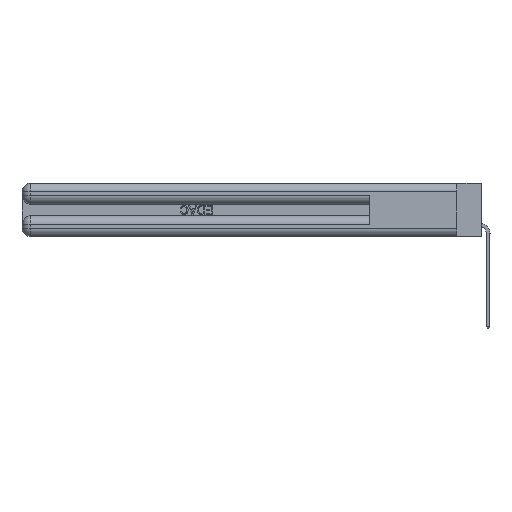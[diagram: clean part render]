
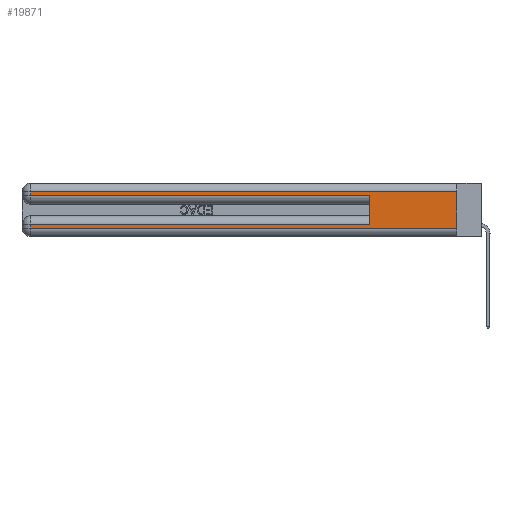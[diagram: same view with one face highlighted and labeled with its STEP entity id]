
A CAD part, left-side view. The second image highlights one B-rep face of the part: STEP entity #19871.
In plain terms, the highlighted planar face has unit normal (-1, 0, 0).
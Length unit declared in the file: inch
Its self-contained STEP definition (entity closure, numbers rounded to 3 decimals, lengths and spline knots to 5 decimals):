
#393 = FACE_OUTER_BOUND ( 'NONE', #48717, .T. ) ;
#705 = DIRECTION ( 'NONE',  ( 0., 0., -1. ) ) ;
#800 = CARTESIAN_POINT ( 'NONE',  ( 0., 0., 0.31 ) ) ;
#820 = CARTESIAN_POINT ( 'NONE',  ( 0., 2.94, 0.085 ) ) ;
#1202 = DIRECTION ( 'NONE',  ( 0., -1., 0. ) ) ;
#2137 = CARTESIAN_POINT ( 'NONE',  ( 0., 0.6, 0.145 ) ) ;
#3164 = LINE ( 'NONE', #20812, #43230 ) ;
#6102 = EDGE_CURVE ( 'NONE', #22808, #16744, #39163, .T. ) ;
#6666 = CARTESIAN_POINT ( 'NONE',  ( 0., 0.6, 0.085 ) ) ;
#9406 = LINE ( 'NONE', #800, #34781 ) ;
#10379 = DIRECTION ( 'NONE',  ( 0., 0., 1. ) ) ;
#10628 = VERTEX_POINT ( 'NONE', #6666 ) ;
#11067 = CARTESIAN_POINT ( 'NONE',  ( 0., 0., 0.06 ) ) ;
#11150 = VERTEX_POINT ( 'NONE', #13514 ) ;
#11471 = VECTOR ( 'NONE', #31491, 39.37008 ) ;
#12427 = ORIENTED_EDGE ( 'NONE', *, *, #43336, .T. ) ;
#12521 = DIRECTION ( 'NONE',  ( 0., 1., 0. ) ) ;
#12815 = VERTEX_POINT ( 'NONE', #41090 ) ;
#13514 = CARTESIAN_POINT ( 'NONE',  ( 0., 0., 0.06 ) ) ;
#13626 = DIRECTION ( 'NONE',  ( 0., 0., -1. ) ) ;
#14155 = VERTEX_POINT ( 'NONE', #41047 ) ;
#14516 = CARTESIAN_POINT ( 'NONE',  ( 0., 0., 0.085 ) ) ;
#16612 = CARTESIAN_POINT ( 'NONE',  ( 0., 2.94, 0.285 ) ) ;
#16744 = VERTEX_POINT ( 'NONE', #16612 ) ;
#17571 = ORIENTED_EDGE ( 'NONE', *, *, #6102, .T. ) ;
#17596 = EDGE_CURVE ( 'NONE', #12815, #11150, #41905, .T. ) ;
#19658 = VERTEX_POINT ( 'NONE', #820 ) ;
#19871 = ADVANCED_FACE ( 'NONE', ( #393 ), #37093, .F. ) ;
#20070 = EDGE_CURVE ( 'NONE', #19658, #14155, #26287, .T. ) ;
#20812 = CARTESIAN_POINT ( 'NONE',  ( 0., 0., 0.285 ) ) ;
#22075 = EDGE_CURVE ( 'NONE', #10628, #43003, #44084, .T. ) ;
#22808 = VERTEX_POINT ( 'NONE', #40728 ) ;
#23227 = LINE ( 'NONE', #11067, #11471 ) ;
#25273 = VECTOR ( 'NONE', #30779, 39.37008 ) ;
#25377 = AXIS2_PLACEMENT_3D ( 'NONE', #49376, #46627, #34970 ) ;
#26287 = LINE ( 'NONE', #43594, #35593 ) ;
#27361 = VECTOR ( 'NONE', #13626, 39.37008 ) ;
#28286 = CARTESIAN_POINT ( 'NONE',  ( 0., 0.6, 0.285 ) ) ;
#28544 = DIRECTION ( 'NONE',  ( 0., 0., -1. ) ) ;
#29983 = ORIENTED_EDGE ( 'NONE', *, *, #34558, .T. ) ;
#30628 = ORIENTED_EDGE ( 'NONE', *, *, #32607, .T. ) ;
#30713 = VECTOR ( 'NONE', #28544, 39.37008 ) ;
#30779 = DIRECTION ( 'NONE',  ( 0., 1., 0. ) ) ;
#31491 = DIRECTION ( 'NONE',  ( 0., -1., 0. ) ) ;
#31567 = ORIENTED_EDGE ( 'NONE', *, *, #45541, .T. ) ;
#32607 = EDGE_CURVE ( 'NONE', #10628, #19658, #50708, .T. ) ;
#33858 = CARTESIAN_POINT ( 'NONE',  ( 0., 2.94, 0.37 ) ) ;
#34558 = EDGE_CURVE ( 'NONE', #14155, #11150, #23227, .T. ) ;
#34781 = VECTOR ( 'NONE', #12521, 39.37008 ) ;
#34970 = DIRECTION ( 'NONE',  ( 0., 0., -1. ) ) ;
#35139 = ORIENTED_EDGE ( 'NONE', *, *, #22075, .F. ) ;
#35593 = VECTOR ( 'NONE', #705, 39.37008 ) ;
#35951 = ORIENTED_EDGE ( 'NONE', *, *, #17596, .F. ) ;
#37093 = PLANE ( 'NONE',  #25377 ) ;
#37314 = ORIENTED_EDGE ( 'NONE', *, *, #20070, .T. ) ;
#39163 = LINE ( 'NONE', #33858, #27361 ) ;
#40189 = CARTESIAN_POINT ( 'NONE',  ( 0., 0., 0.37 ) ) ;
#40728 = CARTESIAN_POINT ( 'NONE',  ( 0., 2.94, 0.31 ) ) ;
#41012 = VECTOR ( 'NONE', #10379, 39.37008 ) ;
#41047 = CARTESIAN_POINT ( 'NONE',  ( 0., 2.94, 0.06 ) ) ;
#41090 = CARTESIAN_POINT ( 'NONE',  ( 0., 0., 0.31 ) ) ;
#41905 = LINE ( 'NONE', #40189, #30713 ) ;
#43003 = VERTEX_POINT ( 'NONE', #28286 ) ;
#43230 = VECTOR ( 'NONE', #1202, 39.37008 ) ;
#43336 = EDGE_CURVE ( 'NONE', #16744, #43003, #3164, .T. ) ;
#43594 = CARTESIAN_POINT ( 'NONE',  ( 0., 2.94, 0.37 ) ) ;
#44084 = LINE ( 'NONE', #2137, #41012 ) ;
#45541 = EDGE_CURVE ( 'NONE', #12815, #22808, #9406, .T. ) ;
#46627 = DIRECTION ( 'NONE',  ( 1., 0., 0. ) ) ;
#48717 = EDGE_LOOP ( 'NONE', ( #35951, #31567, #17571, #12427, #35139, #30628, #37314, #29983 ) ) ;
#49376 = CARTESIAN_POINT ( 'NONE',  ( 0., 0., 0.37 ) ) ;
#50708 = LINE ( 'NONE', #14516, #25273 ) ;
